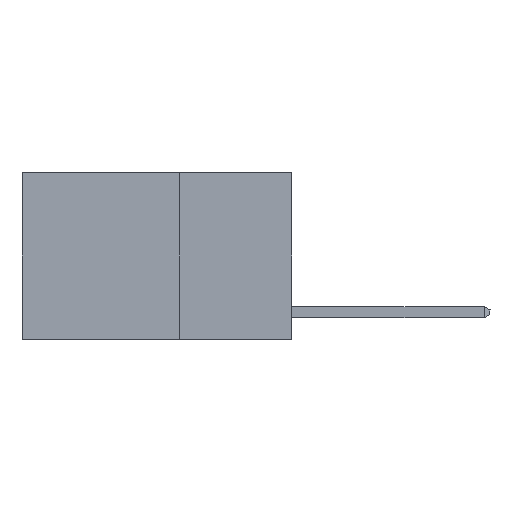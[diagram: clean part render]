
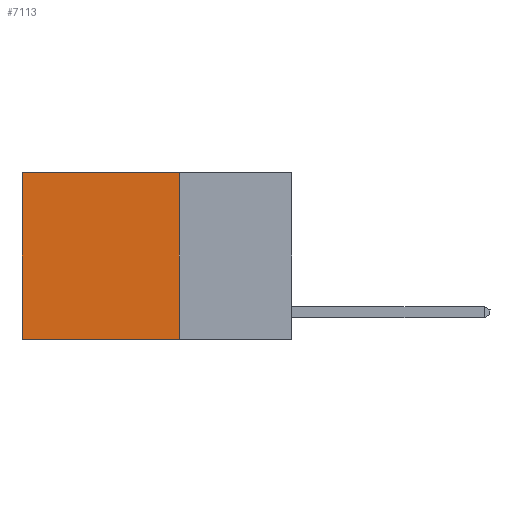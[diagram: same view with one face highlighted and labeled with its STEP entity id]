
A CAD part, left-side view. The second image highlights one B-rep face of the part: STEP entity #7113.
In plain terms, the highlighted planar face has unit normal (-1, 0, 0).
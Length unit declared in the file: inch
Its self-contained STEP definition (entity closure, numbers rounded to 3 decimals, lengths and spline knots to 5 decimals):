
#228 = DIRECTION ( 'NONE',  ( 0., 1., 0. ) ) ;
#312 = CARTESIAN_POINT ( 'NONE',  ( 0.2625, 0.25, 0. ) ) ;
#425 = LINE ( 'NONE', #4627, #9349 ) ;
#1029 = DIRECTION ( 'NONE',  ( 0., 1., 0. ) ) ;
#1046 = DIRECTION ( 'NONE',  ( 1., 0., 0. ) ) ;
#3308 = FACE_OUTER_BOUND ( 'NONE', #9325, .T. ) ;
#3422 = LINE ( 'NONE', #9600, #8260 ) ;
#3435 = CARTESIAN_POINT ( 'NONE',  ( 0.2625, 0.25, 0. ) ) ;
#4570 = PLANE ( 'NONE',  #11204 ) ;
#4627 = CARTESIAN_POINT ( 'NONE',  ( 0.2625, 0.25, -0.37 ) ) ;
#4683 = ORIENTED_EDGE ( 'NONE', *, *, #7831, .T. ) ;
#5131 = ORIENTED_EDGE ( 'NONE', *, *, #9462, .T. ) ;
#5432 = LINE ( 'NONE', #9047, #10708 ) ;
#5485 = DIRECTION ( 'NONE',  ( 0., 0., -1. ) ) ;
#6120 = VERTEX_POINT ( 'NONE', #7156 ) ;
#6224 = VECTOR ( 'NONE', #1029, 39.37008 ) ;
#6850 = DIRECTION ( 'NONE',  ( 0., 0., -1. ) ) ;
#7113 = ADVANCED_FACE ( 'NONE', ( #3308 ), #4570, .F. ) ;
#7156 = CARTESIAN_POINT ( 'NONE',  ( 0.2625, 0.25, -0.37 ) ) ;
#7509 = CARTESIAN_POINT ( 'NONE',  ( 0.2625, 0.25, 0. ) ) ;
#7619 = CARTESIAN_POINT ( 'NONE',  ( 0.2625, 0.6, 0. ) ) ;
#7831 = EDGE_CURVE ( 'NONE', #9046, #9211, #3422, .T. ) ;
#8253 = EDGE_CURVE ( 'NONE', #6120, #9211, #425, .T. ) ;
#8260 = VECTOR ( 'NONE', #5485, 39.37008 ) ;
#8519 = LINE ( 'NONE', #312, #6224 ) ;
#8758 = ORIENTED_EDGE ( 'NONE', *, *, #8794, .F. ) ;
#8794 = EDGE_CURVE ( 'NONE', #11055, #6120, #5432, .T. ) ;
#9046 = VERTEX_POINT ( 'NONE', #7619 ) ;
#9047 = CARTESIAN_POINT ( 'NONE',  ( 0.2625, 0.25, 0. ) ) ;
#9211 = VERTEX_POINT ( 'NONE', #11182 ) ;
#9325 = EDGE_LOOP ( 'NONE', ( #4683, #9664, #8758, #5131 ) ) ;
#9349 = VECTOR ( 'NONE', #228, 39.37008 ) ;
#9462 = EDGE_CURVE ( 'NONE', #11055, #9046, #8519, .T. ) ;
#9600 = CARTESIAN_POINT ( 'NONE',  ( 0.2625, 0.6, 0. ) ) ;
#9664 = ORIENTED_EDGE ( 'NONE', *, *, #8253, .F. ) ;
#10708 = VECTOR ( 'NONE', #10743, 39.37008 ) ;
#10743 = DIRECTION ( 'NONE',  ( 0., 0., -1. ) ) ;
#11055 = VERTEX_POINT ( 'NONE', #7509 ) ;
#11182 = CARTESIAN_POINT ( 'NONE',  ( 0.2625, 0.6, -0.37 ) ) ;
#11204 = AXIS2_PLACEMENT_3D ( 'NONE', #3435, #1046, #6850 ) ;
